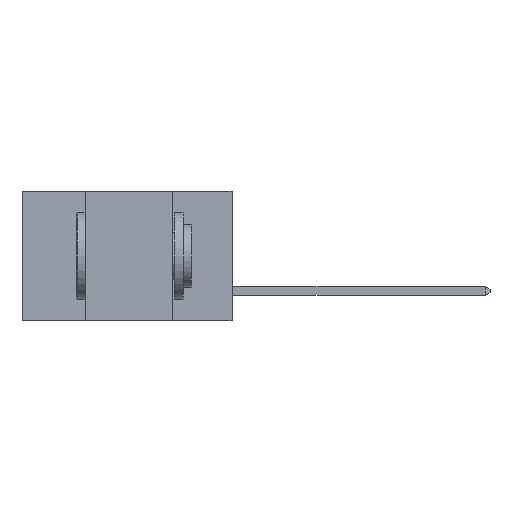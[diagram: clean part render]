
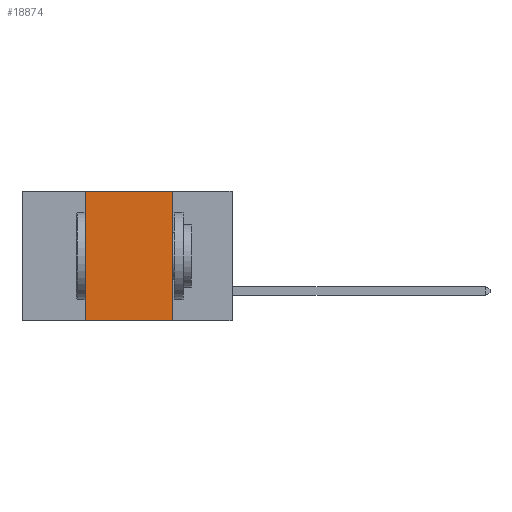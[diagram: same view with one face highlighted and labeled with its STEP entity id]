
A CAD part, left-side view. The second image highlights one B-rep face of the part: STEP entity #18874.
In plain terms, the highlighted planar face has unit normal (-1, 0, 0).
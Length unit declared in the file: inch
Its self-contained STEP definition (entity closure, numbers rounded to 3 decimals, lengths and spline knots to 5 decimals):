
#1686 = VECTOR ( 'NONE', #12905, 39.37008 ) ;
#1816 = DIRECTION ( 'NONE',  ( 1., 0., 0. ) ) ;
#2823 = EDGE_LOOP ( 'NONE', ( #25518, #10571, #26407, #28669 ) ) ;
#3181 = LINE ( 'NONE', #10429, #17774 ) ;
#3716 = VERTEX_POINT ( 'NONE', #25029 ) ;
#4705 = CARTESIAN_POINT ( 'NONE',  ( 0., 0.42, 0. ) ) ;
#6665 = VERTEX_POINT ( 'NONE', #4705 ) ;
#7021 = LINE ( 'NONE', #25330, #21548 ) ;
#7173 = EDGE_CURVE ( 'NONE', #6665, #33337, #3181, .T. ) ;
#8969 = EDGE_CURVE ( 'NONE', #3716, #6665, #13510, .T. ) ;
#10061 = CARTESIAN_POINT ( 'NONE',  ( 0., 0.42, 0. ) ) ;
#10360 = LINE ( 'NONE', #24403, #1686 ) ;
#10429 = CARTESIAN_POINT ( 'NONE',  ( 0., 0.6, 0. ) ) ;
#10494 = PLANE ( 'NONE',  #15656 ) ;
#10571 = ORIENTED_EDGE ( 'NONE', *, *, #7173, .F. ) ;
#12905 = DIRECTION ( 'NONE',  ( 0., -1., 0. ) ) ;
#12997 = DIRECTION ( 'NONE',  ( 0., 0., 1. ) ) ;
#13340 = DIRECTION ( 'NONE',  ( 0., -1., 0. ) ) ;
#13510 = LINE ( 'NONE', #10061, #27961 ) ;
#14275 = FACE_OUTER_BOUND ( 'NONE', #2823, .T. ) ;
#15656 = AXIS2_PLACEMENT_3D ( 'NONE', #19223, #1816, #22133 ) ;
#16866 = EDGE_CURVE ( 'NONE', #3716, #19148, #10360, .T. ) ;
#17774 = VECTOR ( 'NONE', #13340, 39.37008 ) ;
#18260 = EDGE_CURVE ( 'NONE', #33337, #19148, #7021, .T. ) ;
#18485 = CARTESIAN_POINT ( 'NONE',  ( 0., 0.17, 0. ) ) ;
#18874 = ADVANCED_FACE ( 'NONE', ( #14275 ), #10494, .F. ) ;
#19148 = VERTEX_POINT ( 'NONE', #20488 ) ;
#19223 = CARTESIAN_POINT ( 'NONE',  ( 0., 0.6, 0. ) ) ;
#20488 = CARTESIAN_POINT ( 'NONE',  ( 0., 0.17, -0.37 ) ) ;
#21548 = VECTOR ( 'NONE', #28223, 39.37008 ) ;
#22133 = DIRECTION ( 'NONE',  ( 0., 0., -1. ) ) ;
#24403 = CARTESIAN_POINT ( 'NONE',  ( 0., 0.6, -0.37 ) ) ;
#25029 = CARTESIAN_POINT ( 'NONE',  ( 0., 0.42, -0.37 ) ) ;
#25330 = CARTESIAN_POINT ( 'NONE',  ( 0., 0.17, 0. ) ) ;
#25518 = ORIENTED_EDGE ( 'NONE', *, *, #18260, .F. ) ;
#26407 = ORIENTED_EDGE ( 'NONE', *, *, #8969, .F. ) ;
#27961 = VECTOR ( 'NONE', #12997, 39.37008 ) ;
#28223 = DIRECTION ( 'NONE',  ( 0., 0., -1. ) ) ;
#28669 = ORIENTED_EDGE ( 'NONE', *, *, #16866, .T. ) ;
#33337 = VERTEX_POINT ( 'NONE', #18485 ) ;
